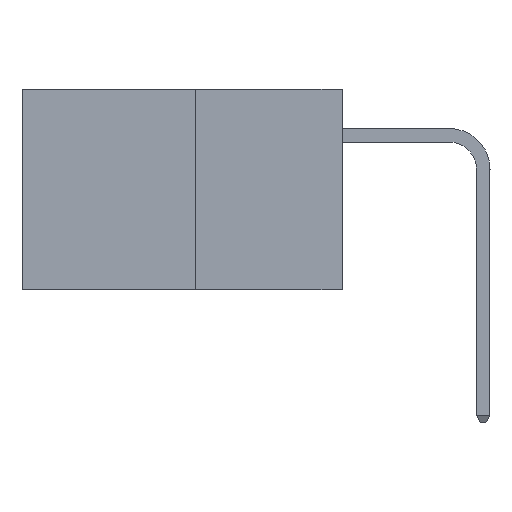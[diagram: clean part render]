
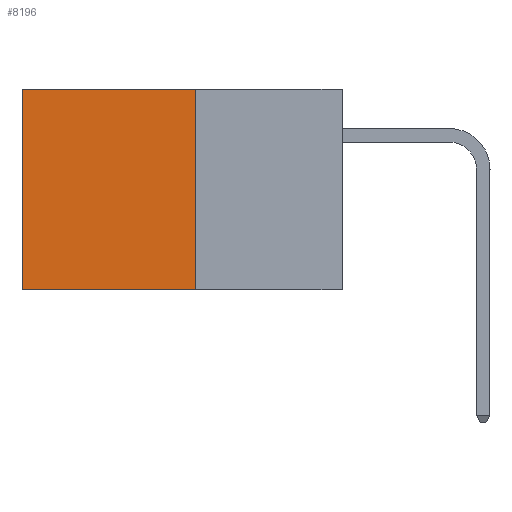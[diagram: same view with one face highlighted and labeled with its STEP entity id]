
A CAD part, left-side view. The second image highlights one B-rep face of the part: STEP entity #8196.
In plain terms, the highlighted planar face has unit normal (-1, 0, 0).
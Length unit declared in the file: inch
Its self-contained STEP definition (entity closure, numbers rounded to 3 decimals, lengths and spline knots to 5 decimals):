
#729 = CARTESIAN_POINT ( 'NONE',  ( 0.277, 0.27, -0.37 ) ) ;
#932 = VERTEX_POINT ( 'NONE', #10225 ) ;
#1075 = CARTESIAN_POINT ( 'NONE',  ( 0.277, 0.59, -0.37 ) ) ;
#1355 = ORIENTED_EDGE ( 'NONE', *, *, #9440, .T. ) ;
#1555 = ORIENTED_EDGE ( 'NONE', *, *, #2363, .F. ) ;
#1573 = DIRECTION ( 'NONE',  ( 0., 1., 0. ) ) ;
#1918 = EDGE_LOOP ( 'NONE', ( #1355, #4118, #1555, #7785 ) ) ;
#2363 = EDGE_CURVE ( 'NONE', #932, #5134, #5599, .T. ) ;
#2727 = EDGE_CURVE ( 'NONE', #5134, #4533, #3441, .T. ) ;
#3441 = LINE ( 'NONE', #729, #8045 ) ;
#3556 = VECTOR ( 'NONE', #3799, 39.37008 ) ;
#3799 = DIRECTION ( 'NONE',  ( 0., 1., 0. ) ) ;
#3823 = LINE ( 'NONE', #9511, #3556 ) ;
#3848 = PLANE ( 'NONE',  #5734 ) ;
#3970 = CARTESIAN_POINT ( 'NONE',  ( 0.277, 0.27, -0.37 ) ) ;
#4118 = ORIENTED_EDGE ( 'NONE', *, *, #2727, .F. ) ;
#4460 = LINE ( 'NONE', #6163, #6754 ) ;
#4530 = EDGE_CURVE ( 'NONE', #932, #10096, #3823, .T. ) ;
#4533 = VERTEX_POINT ( 'NONE', #1075 ) ;
#5134 = VERTEX_POINT ( 'NONE', #10736 ) ;
#5566 = DIRECTION ( 'NONE',  ( 0., 0., -1. ) ) ;
#5599 = LINE ( 'NONE', #3970, #7933 ) ;
#5734 = AXIS2_PLACEMENT_3D ( 'NONE', #7277, #10659, #5566 ) ;
#6163 = CARTESIAN_POINT ( 'NONE',  ( 0.277, 0.59, -0.37 ) ) ;
#6754 = VECTOR ( 'NONE', #10394, 39.37008 ) ;
#6973 = FACE_OUTER_BOUND ( 'NONE', #1918, .T. ) ;
#7277 = CARTESIAN_POINT ( 'NONE',  ( 0.277, 0.27, -0.37 ) ) ;
#7785 = ORIENTED_EDGE ( 'NONE', *, *, #4530, .T. ) ;
#7933 = VECTOR ( 'NONE', #8406, 39.37008 ) ;
#8045 = VECTOR ( 'NONE', #1573, 39.37008 ) ;
#8196 = ADVANCED_FACE ( 'NONE', ( #6973 ), #3848, .F. ) ;
#8406 = DIRECTION ( 'NONE',  ( 0., 0., -1. ) ) ;
#9440 = EDGE_CURVE ( 'NONE', #10096, #4533, #4460, .T. ) ;
#9511 = CARTESIAN_POINT ( 'NONE',  ( 0.277, 0.27, 0. ) ) ;
#10096 = VERTEX_POINT ( 'NONE', #10381 ) ;
#10225 = CARTESIAN_POINT ( 'NONE',  ( 0.277, 0.27, 0. ) ) ;
#10381 = CARTESIAN_POINT ( 'NONE',  ( 0.277, 0.59, 0. ) ) ;
#10394 = DIRECTION ( 'NONE',  ( 0., 0., -1. ) ) ;
#10659 = DIRECTION ( 'NONE',  ( 1., 0., 0. ) ) ;
#10736 = CARTESIAN_POINT ( 'NONE',  ( 0.277, 0.27, -0.37 ) ) ;
